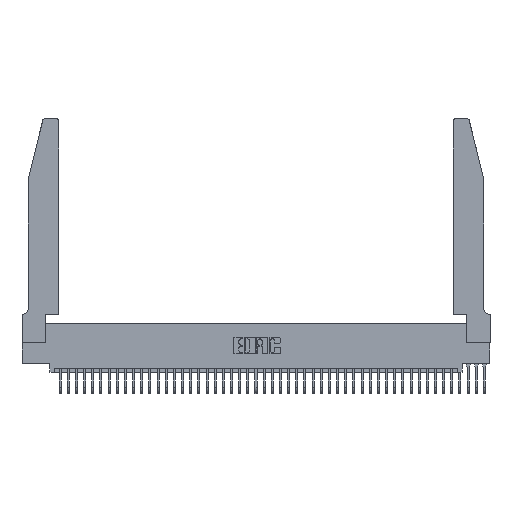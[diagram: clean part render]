
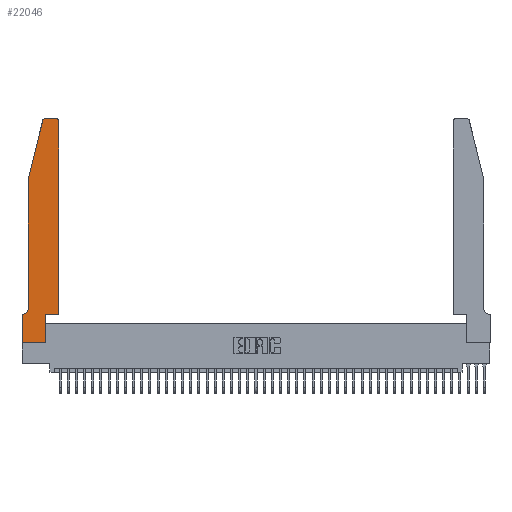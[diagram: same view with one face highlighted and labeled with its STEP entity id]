
A CAD part, top view. The second image highlights one B-rep face of the part: STEP entity #22046.
In plain terms, the highlighted planar face has unit normal (0, 0, 1).
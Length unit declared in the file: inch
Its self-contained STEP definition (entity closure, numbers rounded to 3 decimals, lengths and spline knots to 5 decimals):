
#170 = VECTOR ( 'NONE', #4213, 39.37008 ) ;
#385 = EDGE_CURVE ( 'NONE', #6481, #6596, #28545, .T. ) ;
#580 = ORIENTED_EDGE ( 'NONE', *, *, #26574, .T. ) ;
#583 = CARTESIAN_POINT ( 'NONE',  ( 0.2605, 2.75, 0.37 ) ) ;
#842 = LINE ( 'NONE', #11053, #33033 ) ;
#1340 = FACE_OUTER_BOUND ( 'NONE', #39374, .T. ) ;
#2808 = VECTOR ( 'NONE', #3849, 39.37008 ) ;
#2965 = DIRECTION ( 'NONE',  ( -0.239, -0.971, 0. ) ) ;
#3475 = CIRCLE ( 'NONE', #32389, 0.07 ) ;
#3674 = ORIENTED_EDGE ( 'NONE', *, *, #20330, .T. ) ;
#3757 = CARTESIAN_POINT ( 'NONE',  ( 0.284, 2.72, 0.37 ) ) ;
#3814 = VECTOR ( 'NONE', #30758, 39.37008 ) ;
#3849 = DIRECTION ( 'NONE',  ( -1., 0., 0. ) ) ;
#4213 = DIRECTION ( 'NONE',  ( 0., -1., 0. ) ) ;
#4901 = VECTOR ( 'NONE', #36041, 39.37008 ) ;
#5704 = CARTESIAN_POINT ( 'NONE',  ( 0.4505, 0.35, 0.37 ) ) ;
#6000 = CARTESIAN_POINT ( 'NONE',  ( 0.284, 2.75, 0.37 ) ) ;
#6342 = EDGE_CURVE ( 'NONE', #11094, #30428, #34291, .T. ) ;
#6481 = VERTEX_POINT ( 'NONE', #36785 ) ;
#6596 = VERTEX_POINT ( 'NONE', #40165 ) ;
#6647 = DIRECTION ( 'NONE',  ( 0., 0., 1. ) ) ;
#6985 = DIRECTION ( 'NONE',  ( 1., 0., 0. ) ) ;
#7391 = EDGE_CURVE ( 'NONE', #40084, #20615, #27305, .T. ) ;
#7897 = ORIENTED_EDGE ( 'NONE', *, *, #6342, .T. ) ;
#9349 = DIRECTION ( 'NONE',  ( 0., 0., 1. ) ) ;
#9608 = EDGE_CURVE ( 'NONE', #34368, #17497, #3475, .T. ) ;
#9621 = ORIENTED_EDGE ( 'NONE', *, *, #18854, .T. ) ;
#11053 = CARTESIAN_POINT ( 'NONE',  ( 0.0755, 0.35, 0.37 ) ) ;
#11094 = VERTEX_POINT ( 'NONE', #33616 ) ;
#12223 = ORIENTED_EDGE ( 'NONE', *, *, #25521, .T. ) ;
#12439 = CARTESIAN_POINT ( 'NONE',  ( 0., 0.35, 0.37 ) ) ;
#13162 = CARTESIAN_POINT ( 'NONE',  ( 0.2865, 0.35, 0.37 ) ) ;
#13511 = LINE ( 'NONE', #16974, #4901 ) ;
#13709 = ORIENTED_EDGE ( 'NONE', *, *, #385, .T. ) ;
#13721 = VERTEX_POINT ( 'NONE', #27710 ) ;
#14007 = AXIS2_PLACEMENT_3D ( 'NONE', #12439, #9349, #31762 ) ;
#14418 = VERTEX_POINT ( 'NONE', #6000 ) ;
#14852 = VECTOR ( 'NONE', #16437, 39.37008 ) ;
#15193 = VECTOR ( 'NONE', #29199, 39.37008 ) ;
#15238 = ORIENTED_EDGE ( 'NONE', *, *, #21780, .T. ) ;
#15828 = ORIENTED_EDGE ( 'NONE', *, *, #16098, .T. ) ;
#16098 = EDGE_CURVE ( 'NONE', #14418, #6481, #38499, .T. ) ;
#16437 = DIRECTION ( 'NONE',  ( 0., 1., 0. ) ) ;
#16580 = CARTESIAN_POINT ( 'NONE',  ( 0.0055, 0.42, 0.37 ) ) ;
#16974 = CARTESIAN_POINT ( 'NONE',  ( 0.4505, 0.35, 0.37 ) ) ;
#17497 = VERTEX_POINT ( 'NONE', #39197 ) ;
#18271 = CARTESIAN_POINT ( 'NONE',  ( 0., 0., 0.37 ) ) ;
#18854 = EDGE_CURVE ( 'NONE', #35787, #40084, #31854, .T. ) ;
#19833 = DIRECTION ( 'NONE',  ( -1., 0., 0. ) ) ;
#20330 = EDGE_CURVE ( 'NONE', #30428, #13721, #40213, .T. ) ;
#20615 = VERTEX_POINT ( 'NONE', #27381 ) ;
#20787 = DIRECTION ( 'NONE',  ( -1., 0., 0. ) ) ;
#20878 = CARTESIAN_POINT ( 'NONE',  ( 0.4505, 2.72, 0.37 ) ) ;
#21780 = EDGE_CURVE ( 'NONE', #17497, #11094, #842, .T. ) ;
#21818 = DIRECTION ( 'NONE',  ( 0., 1., 0. ) ) ;
#22046 = ADVANCED_FACE ( 'NONE', ( #1340 ), #28566, .T. ) ;
#23072 = CARTESIAN_POINT ( 'NONE',  ( 0.0755, 0.42, 0.37 ) ) ;
#23377 = VECTOR ( 'NONE', #21818, 39.37008 ) ;
#23536 = CARTESIAN_POINT ( 'NONE',  ( 0.4505, 0.35, 0.37 ) ) ;
#25521 = EDGE_CURVE ( 'NONE', #6596, #34368, #29471, .T. ) ;
#25932 = CARTESIAN_POINT ( 'NONE',  ( 0.4205, 2.72, 0.37 ) ) ;
#26134 = ORIENTED_EDGE ( 'NONE', *, *, #36784, .T. ) ;
#26275 = DIRECTION ( 'NONE',  ( 0., 0., 1. ) ) ;
#26527 = VECTOR ( 'NONE', #2965, 39.37008 ) ;
#26574 = EDGE_CURVE ( 'NONE', #13721, #36080, #39916, .T. ) ;
#27305 = CIRCLE ( 'NONE', #35650, 0.03 ) ;
#27381 = CARTESIAN_POINT ( 'NONE',  ( 0.4205, 2.75, 0.37 ) ) ;
#27554 = ORIENTED_EDGE ( 'NONE', *, *, #9608, .T. ) ;
#27556 = CARTESIAN_POINT ( 'NONE',  ( 0.0755, 2., 0.37 ) ) ;
#27710 = CARTESIAN_POINT ( 'NONE',  ( 0.2865, 0., 0.37 ) ) ;
#28504 = LINE ( 'NONE', #583, #2808 ) ;
#28532 = CARTESIAN_POINT ( 'NONE',  ( 0.2865, 0.35, 0.37 ) ) ;
#28545 = LINE ( 'NONE', #28719, #26527 ) ;
#28566 = PLANE ( 'NONE',  #14007 ) ;
#28719 = CARTESIAN_POINT ( 'NONE',  ( 0.0755, 2., 0.37 ) ) ;
#29160 = DIRECTION ( 'NONE',  ( 1., 0., 0. ) ) ;
#29199 = DIRECTION ( 'NONE',  ( 1., 0., 0. ) ) ;
#29471 = LINE ( 'NONE', #27556, #3814 ) ;
#30428 = VERTEX_POINT ( 'NONE', #18271 ) ;
#30758 = DIRECTION ( 'NONE',  ( 0., -1., 0. ) ) ;
#31762 = DIRECTION ( 'NONE',  ( 1., 0., 0. ) ) ;
#31854 = LINE ( 'NONE', #5704, #23377 ) ;
#32389 = AXIS2_PLACEMENT_3D ( 'NONE', #16580, #38575, #19833 ) ;
#32399 = CARTESIAN_POINT ( 'NONE',  ( 0., 0., 0.37 ) ) ;
#33033 = VECTOR ( 'NONE', #20787, 39.37008 ) ;
#33107 = CARTESIAN_POINT ( 'NONE',  ( 0., 0., 0.37 ) ) ;
#33616 = CARTESIAN_POINT ( 'NONE',  ( 0., 0.35, 0.37 ) ) ;
#33858 = ORIENTED_EDGE ( 'NONE', *, *, #35751, .T. ) ;
#34291 = LINE ( 'NONE', #33107, #170 ) ;
#34368 = VERTEX_POINT ( 'NONE', #23072 ) ;
#34661 = AXIS2_PLACEMENT_3D ( 'NONE', #3757, #26275, #6985 ) ;
#35650 = AXIS2_PLACEMENT_3D ( 'NONE', #25932, #6647, #29160 ) ;
#35751 = EDGE_CURVE ( 'NONE', #36080, #35787, #13511, .T. ) ;
#35787 = VERTEX_POINT ( 'NONE', #23536 ) ;
#36041 = DIRECTION ( 'NONE',  ( 1., 0., 0. ) ) ;
#36080 = VERTEX_POINT ( 'NONE', #28532 ) ;
#36543 = ORIENTED_EDGE ( 'NONE', *, *, #7391, .T. ) ;
#36784 = EDGE_CURVE ( 'NONE', #20615, #14418, #28504, .T. ) ;
#36785 = CARTESIAN_POINT ( 'NONE',  ( 0.25487, 2.72718, 0.37 ) ) ;
#38499 = CIRCLE ( 'NONE', #34661, 0.03 ) ;
#38575 = DIRECTION ( 'NONE',  ( 0., 0., -1. ) ) ;
#39197 = CARTESIAN_POINT ( 'NONE',  ( 0.0055, 0.35, 0.37 ) ) ;
#39374 = EDGE_LOOP ( 'NONE', ( #26134, #15828, #13709, #12223, #27554, #15238, #7897, #3674, #580, #33858, #9621, #36543 ) ) ;
#39916 = LINE ( 'NONE', #13162, #14852 ) ;
#40084 = VERTEX_POINT ( 'NONE', #20878 ) ;
#40165 = CARTESIAN_POINT ( 'NONE',  ( 0.0755, 2., 0.37 ) ) ;
#40213 = LINE ( 'NONE', #32399, #15193 ) ;
